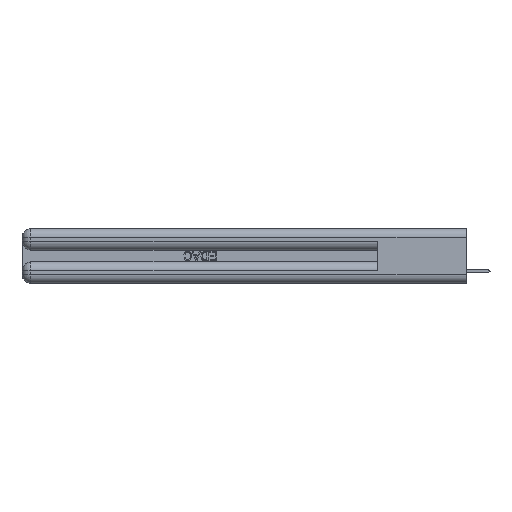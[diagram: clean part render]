
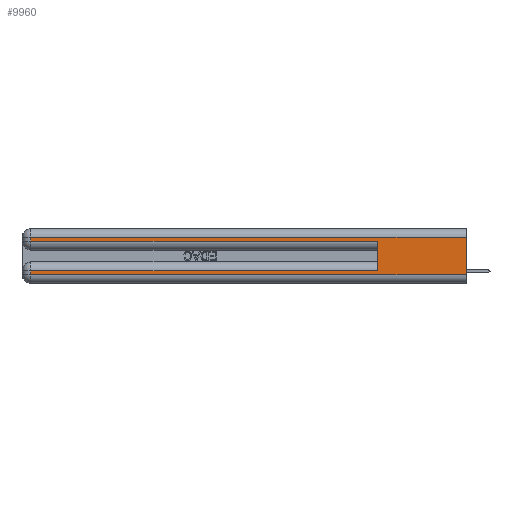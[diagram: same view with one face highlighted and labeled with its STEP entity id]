
A CAD part, left-side view. The second image highlights one B-rep face of the part: STEP entity #9960.
In plain terms, the highlighted planar face has unit normal (-1, 0, 0).
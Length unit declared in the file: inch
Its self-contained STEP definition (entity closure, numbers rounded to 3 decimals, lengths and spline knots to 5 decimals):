
#435 = LINE ( 'NONE', #37605, #1088 ) ;
#1088 = VECTOR ( 'NONE', #4082, 39.37008 ) ;
#1723 = CARTESIAN_POINT ( 'NONE',  ( 0., 0., 0.06 ) ) ;
#2009 = AXIS2_PLACEMENT_3D ( 'NONE', #7488, #14461, #22406 ) ;
#3140 = LINE ( 'NONE', #28060, #35429 ) ;
#4082 = DIRECTION ( 'NONE',  ( 0., 0., 1. ) ) ;
#4346 = VERTEX_POINT ( 'NONE', #25068 ) ;
#4686 = VECTOR ( 'NONE', #22774, 39.37008 ) ;
#4938 = PLANE ( 'NONE',  #2009 ) ;
#4994 = ORIENTED_EDGE ( 'NONE', *, *, #18095, .T. ) ;
#5626 = EDGE_CURVE ( 'NONE', #4346, #12386, #19447, .T. ) ;
#5971 = EDGE_CURVE ( 'NONE', #12386, #14929, #27654, .T. ) ;
#6677 = DIRECTION ( 'NONE',  ( 0., 0., -1. ) ) ;
#7488 = CARTESIAN_POINT ( 'NONE',  ( 0., 0., 0.37 ) ) ;
#7868 = VERTEX_POINT ( 'NONE', #8612 ) ;
#8225 = EDGE_LOOP ( 'NONE', ( #40195, #4994, #45049, #21344, #38690, #32688, #41590, #39270 ) ) ;
#8273 = CARTESIAN_POINT ( 'NONE',  ( 0., 2.94, 0.31 ) ) ;
#8612 = CARTESIAN_POINT ( 'NONE',  ( 0., 0.6, 0.285 ) ) ;
#9500 = VECTOR ( 'NONE', #14007, 39.37008 ) ;
#9960 = ADVANCED_FACE ( 'NONE', ( #38989 ), #4938, .F. ) ;
#10123 = LINE ( 'NONE', #29186, #47615 ) ;
#10175 = CARTESIAN_POINT ( 'NONE',  ( 0., 2.94, 0.37 ) ) ;
#11916 = VECTOR ( 'NONE', #13428, 39.37008 ) ;
#12386 = VERTEX_POINT ( 'NONE', #33878 ) ;
#13428 = DIRECTION ( 'NONE',  ( 0., 0., -1. ) ) ;
#13812 = EDGE_CURVE ( 'NONE', #28312, #7868, #10123, .T. ) ;
#14007 = DIRECTION ( 'NONE',  ( 0., 0., -1. ) ) ;
#14461 = DIRECTION ( 'NONE',  ( 1., 0., 0. ) ) ;
#14898 = EDGE_CURVE ( 'NONE', #17110, #7868, #435, .T. ) ;
#14929 = VERTEX_POINT ( 'NONE', #1723 ) ;
#15567 = CARTESIAN_POINT ( 'NONE',  ( 0., 0., 0.085 ) ) ;
#16726 = CARTESIAN_POINT ( 'NONE',  ( 0., 0., 0.31 ) ) ;
#17110 = VERTEX_POINT ( 'NONE', #36649 ) ;
#17712 = VECTOR ( 'NONE', #38525, 39.37008 ) ;
#18095 = EDGE_CURVE ( 'NONE', #35792, #38663, #3140, .T. ) ;
#18255 = LINE ( 'NONE', #10175, #20619 ) ;
#18339 = CARTESIAN_POINT ( 'NONE',  ( 0., 2.94, 0.285 ) ) ;
#19447 = LINE ( 'NONE', #43451, #9500 ) ;
#20006 = EDGE_CURVE ( 'NONE', #17110, #4346, #39878, .T. ) ;
#20619 = VECTOR ( 'NONE', #6677, 39.37008 ) ;
#21344 = ORIENTED_EDGE ( 'NONE', *, *, #13812, .T. ) ;
#22406 = DIRECTION ( 'NONE',  ( 0., 0., -1. ) ) ;
#22774 = DIRECTION ( 'NONE',  ( 0., 1., 0. ) ) ;
#22831 = EDGE_CURVE ( 'NONE', #38663, #28312, #18255, .T. ) ;
#24007 = CARTESIAN_POINT ( 'NONE',  ( 0., 0., 0.06 ) ) ;
#25068 = CARTESIAN_POINT ( 'NONE',  ( 0., 2.94, 0.085 ) ) ;
#26194 = EDGE_CURVE ( 'NONE', #35792, #14929, #32570, .T. ) ;
#27654 = LINE ( 'NONE', #24007, #17712 ) ;
#28060 = CARTESIAN_POINT ( 'NONE',  ( 0., 0., 0.31 ) ) ;
#28312 = VERTEX_POINT ( 'NONE', #18339 ) ;
#29186 = CARTESIAN_POINT ( 'NONE',  ( 0., 0., 0.285 ) ) ;
#31038 = DIRECTION ( 'NONE',  ( 0., -1., 0. ) ) ;
#32570 = LINE ( 'NONE', #34361, #11916 ) ;
#32688 = ORIENTED_EDGE ( 'NONE', *, *, #20006, .T. ) ;
#33878 = CARTESIAN_POINT ( 'NONE',  ( 0., 2.94, 0.06 ) ) ;
#34361 = CARTESIAN_POINT ( 'NONE',  ( 0., 0., 0.37 ) ) ;
#35429 = VECTOR ( 'NONE', #46220, 39.37008 ) ;
#35792 = VERTEX_POINT ( 'NONE', #16726 ) ;
#36649 = CARTESIAN_POINT ( 'NONE',  ( 0., 0.6, 0.085 ) ) ;
#37605 = CARTESIAN_POINT ( 'NONE',  ( 0., 0.6, 0.145 ) ) ;
#38525 = DIRECTION ( 'NONE',  ( 0., -1., 0. ) ) ;
#38663 = VERTEX_POINT ( 'NONE', #8273 ) ;
#38690 = ORIENTED_EDGE ( 'NONE', *, *, #14898, .F. ) ;
#38989 = FACE_OUTER_BOUND ( 'NONE', #8225, .T. ) ;
#39270 = ORIENTED_EDGE ( 'NONE', *, *, #5971, .T. ) ;
#39878 = LINE ( 'NONE', #15567, #4686 ) ;
#40195 = ORIENTED_EDGE ( 'NONE', *, *, #26194, .F. ) ;
#41590 = ORIENTED_EDGE ( 'NONE', *, *, #5626, .T. ) ;
#43451 = CARTESIAN_POINT ( 'NONE',  ( 0., 2.94, 0.37 ) ) ;
#45049 = ORIENTED_EDGE ( 'NONE', *, *, #22831, .T. ) ;
#46220 = DIRECTION ( 'NONE',  ( 0., 1., 0. ) ) ;
#47615 = VECTOR ( 'NONE', #31038, 39.37008 ) ;
